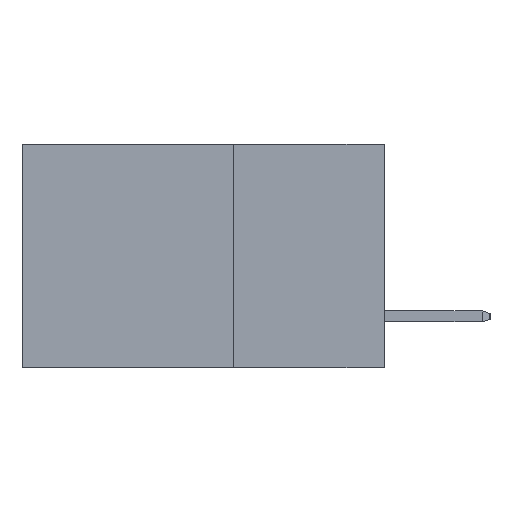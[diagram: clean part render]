
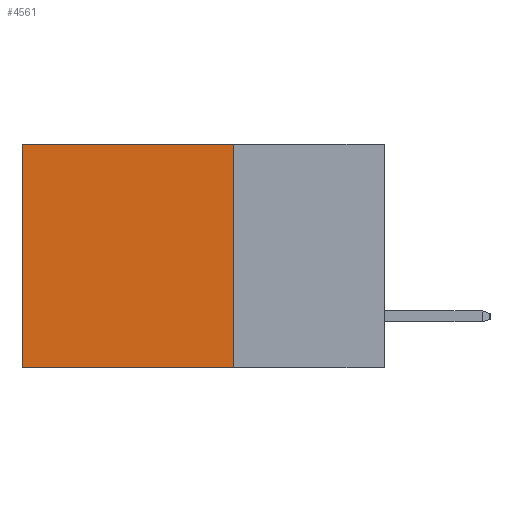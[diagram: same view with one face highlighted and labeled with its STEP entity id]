
A CAD part, left-side view. The second image highlights one B-rep face of the part: STEP entity #4561.
In plain terms, the highlighted planar face has unit normal (-1, 0, 0).
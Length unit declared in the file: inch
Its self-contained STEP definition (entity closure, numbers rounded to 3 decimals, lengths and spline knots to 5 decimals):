
#245 = LINE ( 'NONE', #1599, #13426 ) ;
#589 = CARTESIAN_POINT ( 'NONE',  ( 0.298, 0.6, 0. ) ) ;
#925 = LINE ( 'NONE', #4060, #11789 ) ;
#1326 = ORIENTED_EDGE ( 'NONE', *, *, #5047, .T. ) ;
#1450 = EDGE_LOOP ( 'NONE', ( #1326, #2599, #2567, #4980 ) ) ;
#1599 = CARTESIAN_POINT ( 'NONE',  ( 0.298, 0.25, 0. ) ) ;
#1848 = VERTEX_POINT ( 'NONE', #7771 ) ;
#2567 = ORIENTED_EDGE ( 'NONE', *, *, #11534, .F. ) ;
#2599 = ORIENTED_EDGE ( 'NONE', *, *, #7876, .F. ) ;
#2749 = FACE_OUTER_BOUND ( 'NONE', #1450, .T. ) ;
#3252 = DIRECTION ( 'NONE',  ( 1., 0., 0. ) ) ;
#4060 = CARTESIAN_POINT ( 'NONE',  ( 0.298, 0.25, 0. ) ) ;
#4561 = ADVANCED_FACE ( 'NONE', ( #2749 ), #10365, .F. ) ;
#4969 = VERTEX_POINT ( 'NONE', #11559 ) ;
#4980 = ORIENTED_EDGE ( 'NONE', *, *, #12684, .T. ) ;
#5047 = EDGE_CURVE ( 'NONE', #11471, #10465, #10181, .T. ) ;
#7666 = CARTESIAN_POINT ( 'NONE',  ( 0.298, 0.6, -0.37 ) ) ;
#7771 = CARTESIAN_POINT ( 'NONE',  ( 0.298, 0.25, 0. ) ) ;
#7876 = EDGE_CURVE ( 'NONE', #4969, #10465, #11478, .T. ) ;
#8349 = AXIS2_PLACEMENT_3D ( 'NONE', #12925, #3252, #10099 ) ;
#8450 = DIRECTION ( 'NONE',  ( 0., 1., 0. ) ) ;
#8638 = VECTOR ( 'NONE', #8450, 39.37008 ) ;
#10099 = DIRECTION ( 'NONE',  ( 0., 0., -1. ) ) ;
#10181 = LINE ( 'NONE', #11093, #10792 ) ;
#10349 = DIRECTION ( 'NONE',  ( 0., 0., -1. ) ) ;
#10365 = PLANE ( 'NONE',  #8349 ) ;
#10465 = VERTEX_POINT ( 'NONE', #7666 ) ;
#10792 = VECTOR ( 'NONE', #11208, 39.37008 ) ;
#11093 = CARTESIAN_POINT ( 'NONE',  ( 0.298, 0.6, 0. ) ) ;
#11208 = DIRECTION ( 'NONE',  ( 0., 0., -1. ) ) ;
#11471 = VERTEX_POINT ( 'NONE', #589 ) ;
#11478 = LINE ( 'NONE', #13164, #8638 ) ;
#11534 = EDGE_CURVE ( 'NONE', #1848, #4969, #925, .T. ) ;
#11559 = CARTESIAN_POINT ( 'NONE',  ( 0.298, 0.25, -0.37 ) ) ;
#11789 = VECTOR ( 'NONE', #10349, 39.37008 ) ;
#12073 = DIRECTION ( 'NONE',  ( 0., 1., 0. ) ) ;
#12684 = EDGE_CURVE ( 'NONE', #1848, #11471, #245, .T. ) ;
#12925 = CARTESIAN_POINT ( 'NONE',  ( 0.298, 0.25, 0. ) ) ;
#13164 = CARTESIAN_POINT ( 'NONE',  ( 0.298, 0.25, -0.37 ) ) ;
#13426 = VECTOR ( 'NONE', #12073, 39.37008 ) ;
